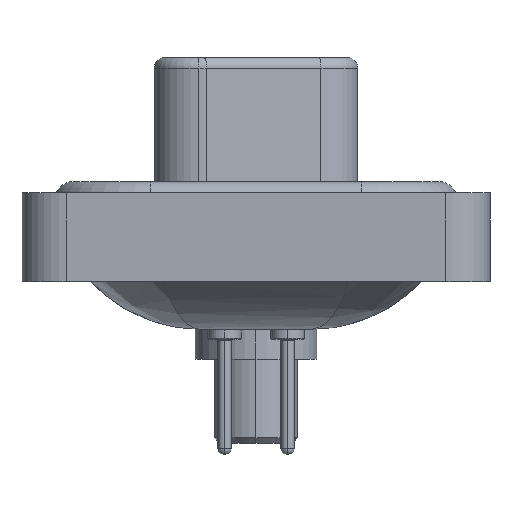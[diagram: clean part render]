
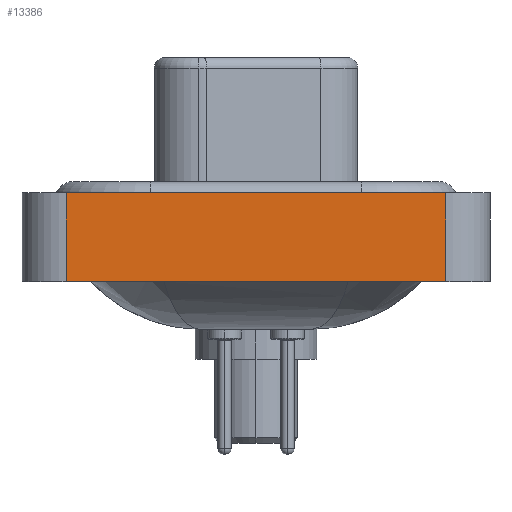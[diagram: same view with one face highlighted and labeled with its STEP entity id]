
A CAD part, left-side view. The second image highlights one B-rep face of the part: STEP entity #13386.
In plain terms, the highlighted planar face has unit normal (-1, 0, 0).
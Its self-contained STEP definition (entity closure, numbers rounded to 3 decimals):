
#263 = VERTEX_POINT ( 'NONE', #716 ) ;
#467 = ORIENTED_EDGE ( 'NONE', *, *, #4942, .T. ) ;
#493 = ORIENTED_EDGE ( 'NONE', *, *, #2074, .F. ) ;
#716 = CARTESIAN_POINT ( 'NONE',  ( -7.25, -8.55, -3.6 ) ) ;
#820 = DIRECTION ( 'NONE',  ( 0., -1., 0. ) ) ;
#2074 = EDGE_CURVE ( 'NONE', #4831, #2276, #10456, .T. ) ;
#2276 = VERTEX_POINT ( 'NONE', #15027 ) ;
#3175 = CARTESIAN_POINT ( 'NONE',  ( -7.25, 8.55, -3.6 ) ) ;
#3512 = PLANE ( 'NONE',  #15316 ) ;
#3616 = EDGE_LOOP ( 'NONE', ( #9375, #9961, #493, #467 ) ) ;
#3804 = EDGE_CURVE ( 'NONE', #263, #8912, #4214, .T. ) ;
#4186 = CARTESIAN_POINT ( 'NONE',  ( -7.25, -8.55, 0.4 ) ) ;
#4214 = LINE ( 'NONE', #9807, #8000 ) ;
#4413 = VECTOR ( 'NONE', #15952, 1000. ) ;
#4831 = VERTEX_POINT ( 'NONE', #3175 ) ;
#4942 = EDGE_CURVE ( 'NONE', #4831, #263, #8939, .T. ) ;
#5130 = CARTESIAN_POINT ( 'NONE',  ( -7.25, -8.55, -3.6 ) ) ;
#6615 = VECTOR ( 'NONE', #8254, 1000. ) ;
#8000 = VECTOR ( 'NONE', #11059, 1000. ) ;
#8254 = DIRECTION ( 'NONE',  ( 0., -1., 0. ) ) ;
#8855 = VECTOR ( 'NONE', #820, 1000. ) ;
#8912 = VERTEX_POINT ( 'NONE', #17320 ) ;
#8939 = LINE ( 'NONE', #17132, #8855 ) ;
#9375 = ORIENTED_EDGE ( 'NONE', *, *, #3804, .T. ) ;
#9807 = CARTESIAN_POINT ( 'NONE',  ( -7.25, -8.55, -3.6 ) ) ;
#9961 = ORIENTED_EDGE ( 'NONE', *, *, #15461, .F. ) ;
#10372 = CARTESIAN_POINT ( 'NONE',  ( -7.25, 8.55, -3.6 ) ) ;
#10456 = LINE ( 'NONE', #10372, #4413 ) ;
#10946 = LINE ( 'NONE', #4186, #6615 ) ;
#11059 = DIRECTION ( 'NONE',  ( 0., 0., 1. ) ) ;
#13386 = ADVANCED_FACE ( 'NONE', ( #17211 ), #3512, .T. ) ;
#14763 = DIRECTION ( 'NONE',  ( -1., 0., 0. ) ) ;
#15027 = CARTESIAN_POINT ( 'NONE',  ( -7.25, 8.55, 0.4 ) ) ;
#15316 = AXIS2_PLACEMENT_3D ( 'NONE', #5130, #14763, #15766 ) ;
#15461 = EDGE_CURVE ( 'NONE', #2276, #8912, #10946, .T. ) ;
#15766 = DIRECTION ( 'NONE',  ( 0., 0., 1. ) ) ;
#15952 = DIRECTION ( 'NONE',  ( 0., 0., 1. ) ) ;
#17132 = CARTESIAN_POINT ( 'NONE',  ( -7.25, -8.55, -3.6 ) ) ;
#17211 = FACE_OUTER_BOUND ( 'NONE', #3616, .T. ) ;
#17320 = CARTESIAN_POINT ( 'NONE',  ( -7.25, -8.55, 0.4 ) ) ;
